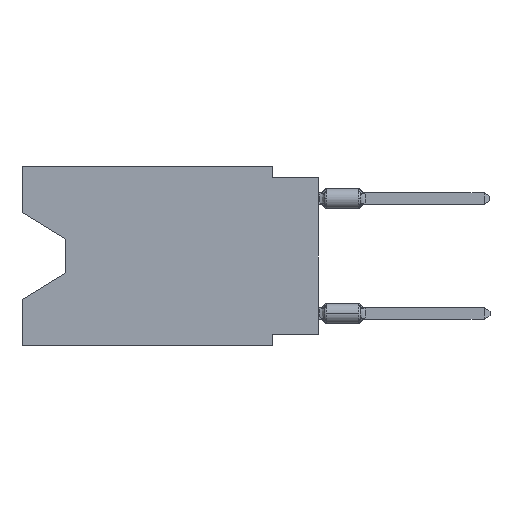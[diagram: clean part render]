
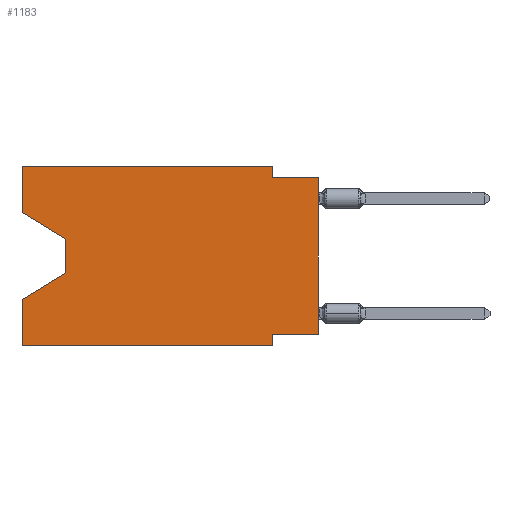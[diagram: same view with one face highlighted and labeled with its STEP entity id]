
A CAD part, left-side view. The second image highlights one B-rep face of the part: STEP entity #1183.
In plain terms, the highlighted planar face has unit normal (-1, 0, 0).
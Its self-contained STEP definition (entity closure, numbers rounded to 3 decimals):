
#228 = LINE ( 'NONE', #21714, #1763 ) ;
#744 = CARTESIAN_POINT ( 'NONE',  ( 0., 16.383, 0. ) ) ;
#1119 = VERTEX_POINT ( 'NONE', #18710 ) ;
#1183 = ADVANCED_FACE ( 'NONE', ( #24807 ), #22615, .F. ) ;
#1382 = CARTESIAN_POINT ( 'NONE',  ( 0., 16.383, -2.546 ) ) ;
#1469 = ORIENTED_EDGE ( 'NONE', *, *, #14371, .T. ) ;
#1528 = EDGE_CURVE ( 'NONE', #15850, #1119, #14708, .T. ) ;
#1645 = DIRECTION ( 'NONE',  ( 0., -0.855, -0.519 ) ) ;
#1763 = VECTOR ( 'NONE', #12273, 1000. ) ;
#1811 = LINE ( 'NONE', #11505, #10155 ) ;
#2036 = CARTESIAN_POINT ( 'NONE',  ( 0., 2.54, 0. ) ) ;
#2374 = EDGE_CURVE ( 'NONE', #10128, #4112, #16448, .T. ) ;
#3027 = VECTOR ( 'NONE', #1645, 1000. ) ;
#4012 = ORIENTED_EDGE ( 'NONE', *, *, #21276, .T. ) ;
#4112 = VERTEX_POINT ( 'NONE', #16926 ) ;
#4539 = AXIS2_PLACEMENT_3D ( 'NONE', #744, #7076, #24428 ) ;
#4781 = VECTOR ( 'NONE', #13380, 1000. ) ;
#4882 = VERTEX_POINT ( 'NONE', #8015 ) ;
#6612 = DIRECTION ( 'NONE',  ( 0., 0.855, -0.519 ) ) ;
#6697 = VECTOR ( 'NONE', #13482, 1000. ) ;
#7076 = DIRECTION ( 'NONE',  ( 1., 0., 0. ) ) ;
#7189 = CARTESIAN_POINT ( 'NONE',  ( 0., 0., -9.271 ) ) ;
#7366 = VERTEX_POINT ( 'NONE', #15961 ) ;
#7438 = CARTESIAN_POINT ( 'NONE',  ( 0., 16.383, -9.906 ) ) ;
#7833 = ORIENTED_EDGE ( 'NONE', *, *, #23881, .F. ) ;
#8015 = CARTESIAN_POINT ( 'NONE',  ( 0., 2.54, -9.271 ) ) ;
#8456 = CARTESIAN_POINT ( 'NONE',  ( 0., 13.97, -5.893 ) ) ;
#8620 = CARTESIAN_POINT ( 'NONE',  ( 0., 2.54, -0.635 ) ) ;
#8793 = LINE ( 'NONE', #24717, #21403 ) ;
#9136 = ORIENTED_EDGE ( 'NONE', *, *, #25284, .T. ) ;
#9193 = CARTESIAN_POINT ( 'NONE',  ( 0., 0., -0.635 ) ) ;
#9613 = CARTESIAN_POINT ( 'NONE',  ( 0., 2.54, -9.906 ) ) ;
#9911 = LINE ( 'NONE', #2036, #14767 ) ;
#9957 = VERTEX_POINT ( 'NONE', #7438 ) ;
#10128 = VERTEX_POINT ( 'NONE', #8456 ) ;
#10155 = VECTOR ( 'NONE', #19920, 1000. ) ;
#10643 = LINE ( 'NONE', #22552, #23085 ) ;
#11077 = VERTEX_POINT ( 'NONE', #7189 ) ;
#11429 = LINE ( 'NONE', #9613, #4781 ) ;
#11505 = CARTESIAN_POINT ( 'NONE',  ( 0., 16.383, 0. ) ) ;
#12004 = ORIENTED_EDGE ( 'NONE', *, *, #1528, .F. ) ;
#12273 = DIRECTION ( 'NONE',  ( 0., 1., 0. ) ) ;
#13380 = DIRECTION ( 'NONE',  ( 0., 0., -1. ) ) ;
#13412 = LINE ( 'NONE', #15745, #15927 ) ;
#13420 = LINE ( 'NONE', #1382, #3027 ) ;
#13482 = DIRECTION ( 'NONE',  ( 0., -1., 0. ) ) ;
#14298 = VERTEX_POINT ( 'NONE', #9193 ) ;
#14371 = EDGE_CURVE ( 'NONE', #9957, #18500, #23169, .T. ) ;
#14708 = LINE ( 'NONE', #16381, #23146 ) ;
#14767 = VECTOR ( 'NONE', #17812, 1000. ) ;
#14930 = EDGE_CURVE ( 'NONE', #11077, #4882, #228, .T. ) ;
#15745 = CARTESIAN_POINT ( 'NONE',  ( 0., 0., -0.635 ) ) ;
#15850 = VERTEX_POINT ( 'NONE', #20711 ) ;
#15927 = VECTOR ( 'NONE', #17159, 1000. ) ;
#15961 = CARTESIAN_POINT ( 'NONE',  ( 0., 16.383, -2.546 ) ) ;
#16263 = CARTESIAN_POINT ( 'NONE',  ( 0., 2.54, -9.906 ) ) ;
#16381 = CARTESIAN_POINT ( 'NONE',  ( 0., 16.383, 0. ) ) ;
#16448 = LINE ( 'NONE', #20586, #17408 ) ;
#16926 = CARTESIAN_POINT ( 'NONE',  ( 0., 16.383, -7.36 ) ) ;
#17081 = EDGE_CURVE ( 'NONE', #25545, #14298, #13412, .T. ) ;
#17159 = DIRECTION ( 'NONE',  ( 0., -1., 0. ) ) ;
#17408 = VECTOR ( 'NONE', #6612, 1000. ) ;
#17613 = CARTESIAN_POINT ( 'NONE',  ( 0., 16.383, -9.906 ) ) ;
#17812 = DIRECTION ( 'NONE',  ( 0., 0., -1. ) ) ;
#17893 = EDGE_CURVE ( 'NONE', #18842, #10128, #23788, .T. ) ;
#18500 = VERTEX_POINT ( 'NONE', #16263 ) ;
#18710 = CARTESIAN_POINT ( 'NONE',  ( 0., 2.54, 0. ) ) ;
#18842 = VERTEX_POINT ( 'NONE', #19979 ) ;
#18873 = DIRECTION ( 'NONE',  ( 0., 0., 1. ) ) ;
#19030 = EDGE_CURVE ( 'NONE', #9957, #4112, #10643, .T. ) ;
#19147 = ORIENTED_EDGE ( 'NONE', *, *, #14930, .F. ) ;
#19398 = CARTESIAN_POINT ( 'NONE',  ( 0., 13.97, -4.013 ) ) ;
#19906 = DIRECTION ( 'NONE',  ( 0., 0., -1. ) ) ;
#19920 = DIRECTION ( 'NONE',  ( 0., 0., 1. ) ) ;
#19979 = CARTESIAN_POINT ( 'NONE',  ( 0., 13.97, -4.013 ) ) ;
#19994 = ORIENTED_EDGE ( 'NONE', *, *, #17893, .T. ) ;
#20586 = CARTESIAN_POINT ( 'NONE',  ( 0., 13.97, -5.893 ) ) ;
#20619 = DIRECTION ( 'NONE',  ( 0., 0., 1. ) ) ;
#20711 = CARTESIAN_POINT ( 'NONE',  ( 0., 16.383, 0. ) ) ;
#20769 = DIRECTION ( 'NONE',  ( 0., -1., 0. ) ) ;
#20924 = ORIENTED_EDGE ( 'NONE', *, *, #23080, .F. ) ;
#20930 = ORIENTED_EDGE ( 'NONE', *, *, #19030, .F. ) ;
#21276 = EDGE_CURVE ( 'NONE', #11077, #14298, #8793, .T. ) ;
#21403 = VECTOR ( 'NONE', #18873, 1000. ) ;
#21682 = EDGE_CURVE ( 'NONE', #4882, #18500, #11429, .T. ) ;
#21714 = CARTESIAN_POINT ( 'NONE',  ( 0., 0., -9.271 ) ) ;
#21722 = EDGE_LOOP ( 'NONE', ( #9136, #19994, #23352, #20930, #1469, #23509, #19147, #4012, #22120, #20924, #12004, #7833 ) ) ;
#22120 = ORIENTED_EDGE ( 'NONE', *, *, #17081, .F. ) ;
#22141 = VECTOR ( 'NONE', #19906, 1000. ) ;
#22552 = CARTESIAN_POINT ( 'NONE',  ( 0., 16.383, 0. ) ) ;
#22615 = PLANE ( 'NONE',  #4539 ) ;
#23080 = EDGE_CURVE ( 'NONE', #1119, #25545, #9911, .T. ) ;
#23085 = VECTOR ( 'NONE', #20619, 1000. ) ;
#23146 = VECTOR ( 'NONE', #20769, 1000. ) ;
#23169 = LINE ( 'NONE', #17613, #6697 ) ;
#23352 = ORIENTED_EDGE ( 'NONE', *, *, #2374, .T. ) ;
#23509 = ORIENTED_EDGE ( 'NONE', *, *, #21682, .F. ) ;
#23788 = LINE ( 'NONE', #19398, #22141 ) ;
#23881 = EDGE_CURVE ( 'NONE', #7366, #15850, #1811, .T. ) ;
#24428 = DIRECTION ( 'NONE',  ( 0., 0., -1. ) ) ;
#24717 = CARTESIAN_POINT ( 'NONE',  ( 0., 0., 0. ) ) ;
#24807 = FACE_OUTER_BOUND ( 'NONE', #21722, .T. ) ;
#25284 = EDGE_CURVE ( 'NONE', #7366, #18842, #13420, .T. ) ;
#25545 = VERTEX_POINT ( 'NONE', #8620 ) ;
